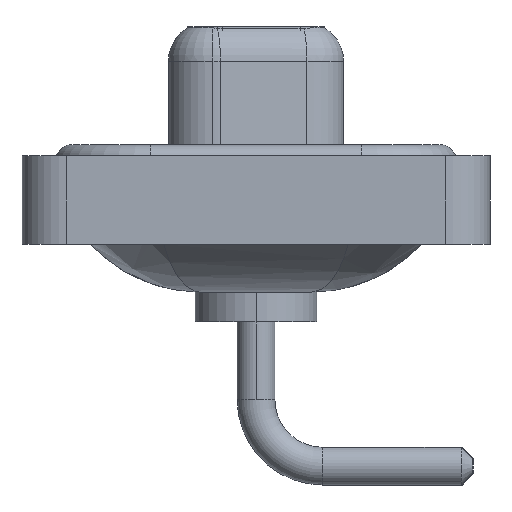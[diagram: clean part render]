
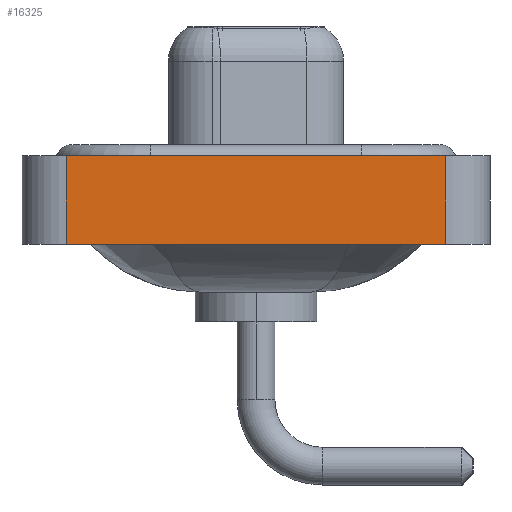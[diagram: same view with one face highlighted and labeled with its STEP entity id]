
A CAD part, left-side view. The second image highlights one B-rep face of the part: STEP entity #16325.
In plain terms, the highlighted planar face has unit normal (-1, 0, 0).
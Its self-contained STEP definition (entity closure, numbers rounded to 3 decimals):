
#722 = VECTOR ( 'NONE', #2748, 1000. ) ;
#753 = DIRECTION ( 'NONE',  ( 0., 0., 1. ) ) ;
#963 = FACE_OUTER_BOUND ( 'NONE', #5355, .T. ) ;
#2243 = PLANE ( 'NONE',  #10522 ) ;
#2748 = DIRECTION ( 'NONE',  ( 0., 0., 1. ) ) ;
#3643 = VECTOR ( 'NONE', #8434, 1000. ) ;
#5245 = CARTESIAN_POINT ( 'NONE',  ( -7.25, -8.55, 0.4 ) ) ;
#5355 = EDGE_LOOP ( 'NONE', ( #7829, #10647, #8755, #8564 ) ) ;
#5859 = LINE ( 'NONE', #9790, #10909 ) ;
#6586 = CARTESIAN_POINT ( 'NONE',  ( -7.25, 8.55, -3.6 ) ) ;
#6734 = EDGE_CURVE ( 'NONE', #12541, #14146, #11573, .T. ) ;
#6874 = CARTESIAN_POINT ( 'NONE',  ( -7.25, -8.55, 0.4 ) ) ;
#7794 = LINE ( 'NONE', #6586, #722 ) ;
#7829 = ORIENTED_EDGE ( 'NONE', *, *, #12719, .T. ) ;
#7907 = DIRECTION ( 'NONE',  ( 0., -1., 0. ) ) ;
#8255 = CARTESIAN_POINT ( 'NONE',  ( -7.25, 8.55, 0.4 ) ) ;
#8434 = DIRECTION ( 'NONE',  ( 0., -1., 0. ) ) ;
#8510 = CARTESIAN_POINT ( 'NONE',  ( -7.25, -8.55, -3.6 ) ) ;
#8564 = ORIENTED_EDGE ( 'NONE', *, *, #8910, .T. ) ;
#8755 = ORIENTED_EDGE ( 'NONE', *, *, #16098, .F. ) ;
#8910 = EDGE_CURVE ( 'NONE', #13314, #16139, #12458, .T. ) ;
#9790 = CARTESIAN_POINT ( 'NONE',  ( -7.25, -8.55, -3.6 ) ) ;
#10522 = AXIS2_PLACEMENT_3D ( 'NONE', #15233, #15062, #11194 ) ;
#10647 = ORIENTED_EDGE ( 'NONE', *, *, #6734, .F. ) ;
#10909 = VECTOR ( 'NONE', #753, 1000. ) ;
#11194 = DIRECTION ( 'NONE',  ( 0., 0., 1. ) ) ;
#11573 = LINE ( 'NONE', #5245, #12339 ) ;
#12339 = VECTOR ( 'NONE', #7907, 1000. ) ;
#12458 = LINE ( 'NONE', #8510, #3643 ) ;
#12541 = VERTEX_POINT ( 'NONE', #8255 ) ;
#12719 = EDGE_CURVE ( 'NONE', #16139, #14146, #5859, .T. ) ;
#13314 = VERTEX_POINT ( 'NONE', #15416 ) ;
#13695 = CARTESIAN_POINT ( 'NONE',  ( -7.25, -8.55, -3.6 ) ) ;
#14146 = VERTEX_POINT ( 'NONE', #6874 ) ;
#15062 = DIRECTION ( 'NONE',  ( -1., 0., 0. ) ) ;
#15233 = CARTESIAN_POINT ( 'NONE',  ( -7.25, -8.55, -3.6 ) ) ;
#15416 = CARTESIAN_POINT ( 'NONE',  ( -7.25, 8.55, -3.6 ) ) ;
#16098 = EDGE_CURVE ( 'NONE', #13314, #12541, #7794, .T. ) ;
#16139 = VERTEX_POINT ( 'NONE', #13695 ) ;
#16325 = ADVANCED_FACE ( 'NONE', ( #963 ), #2243, .T. ) ;
